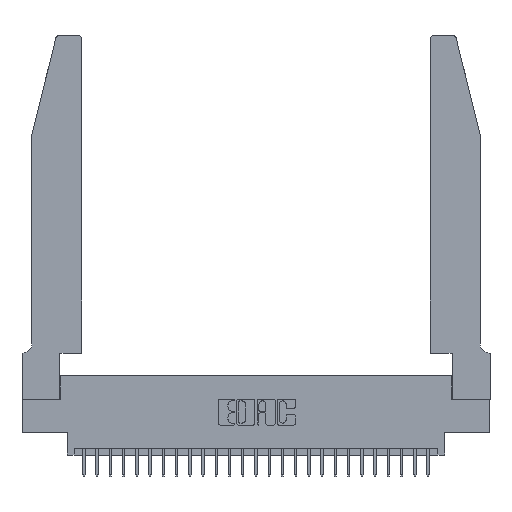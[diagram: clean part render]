
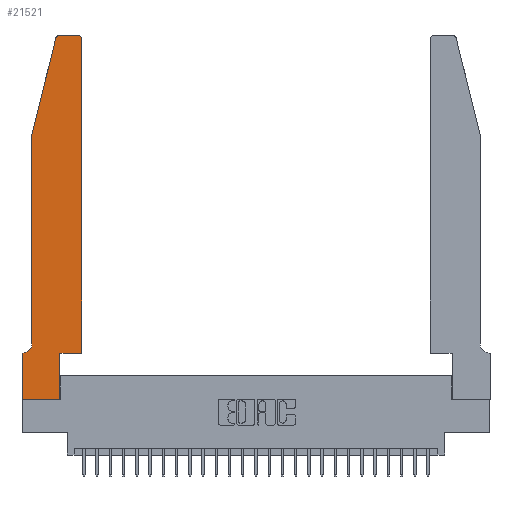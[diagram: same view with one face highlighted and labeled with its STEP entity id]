
A CAD part, top view. The second image highlights one B-rep face of the part: STEP entity #21521.
In plain terms, the highlighted planar face has unit normal (0, 0, 1).
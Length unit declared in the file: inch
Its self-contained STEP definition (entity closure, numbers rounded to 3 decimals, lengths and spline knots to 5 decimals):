
#35 = ORIENTED_EDGE ( 'NONE', *, *, #12355, .T. ) ;
#181 = CIRCLE ( 'NONE', #6082, 0.03 ) ;
#183 = CARTESIAN_POINT ( 'NONE',  ( 0.0755, 0.42, 0.37 ) ) ;
#223 = DIRECTION ( 'NONE',  ( 1., 0., 0. ) ) ;
#316 = CIRCLE ( 'NONE', #5066, 0.03 ) ;
#522 = VERTEX_POINT ( 'NONE', #19357 ) ;
#789 = ORIENTED_EDGE ( 'NONE', *, *, #21840, .T. ) ;
#815 = VECTOR ( 'NONE', #20764, 39.37008 ) ;
#1147 = CIRCLE ( 'NONE', #15072, 0.07 ) ;
#1433 = VECTOR ( 'NONE', #27402, 39.37008 ) ;
#1492 = LINE ( 'NONE', #7889, #815 ) ;
#1853 = CARTESIAN_POINT ( 'NONE',  ( 0.4505, 0.35, 0.37 ) ) ;
#1900 = VERTEX_POINT ( 'NONE', #2422 ) ;
#2214 = PLANE ( 'NONE',  #9395 ) ;
#2422 = CARTESIAN_POINT ( 'NONE',  ( 0.0755, 2., 0.37 ) ) ;
#2505 = DIRECTION ( 'NONE',  ( 0., 0., 1. ) ) ;
#2777 = VECTOR ( 'NONE', #16796, 39.37008 ) ;
#3103 = EDGE_CURVE ( 'NONE', #25998, #522, #1147, .T. ) ;
#3279 = DIRECTION ( 'NONE',  ( -1., 0., 0. ) ) ;
#3479 = DIRECTION ( 'NONE',  ( 1., 0., 0. ) ) ;
#3489 = LINE ( 'NONE', #9904, #1433 ) ;
#3537 = CARTESIAN_POINT ( 'NONE',  ( 0.25487, 2.72718, 0.37 ) ) ;
#3566 = DIRECTION ( 'NONE',  ( 0., 0., 1. ) ) ;
#3893 = LINE ( 'NONE', #26260, #12405 ) ;
#4237 = DIRECTION ( 'NONE',  ( -1., 0., 0. ) ) ;
#4612 = EDGE_CURVE ( 'NONE', #1900, #25998, #3489, .T. ) ;
#4697 = EDGE_CURVE ( 'NONE', #15780, #19619, #20827, .T. ) ;
#5066 = AXIS2_PLACEMENT_3D ( 'NONE', #10025, #3566, #27527 ) ;
#5402 = EDGE_LOOP ( 'NONE', ( #14896, #9479, #789, #10932, #7131, #21754, #7157, #11829, #24147, #20751, #17700, #35 ) ) ;
#5901 = VERTEX_POINT ( 'NONE', #23033 ) ;
#6082 = AXIS2_PLACEMENT_3D ( 'NONE', #6675, #19821, #223 ) ;
#6093 = CARTESIAN_POINT ( 'NONE',  ( 0.0755, 2., 0.37 ) ) ;
#6245 = CARTESIAN_POINT ( 'NONE',  ( 0.2865, 0.35, 0.37 ) ) ;
#6675 = CARTESIAN_POINT ( 'NONE',  ( 0.284, 2.72, 0.37 ) ) ;
#7131 = ORIENTED_EDGE ( 'NONE', *, *, #3103, .T. ) ;
#7157 = ORIENTED_EDGE ( 'NONE', *, *, #9062, .T. ) ;
#7889 = CARTESIAN_POINT ( 'NONE',  ( 0.0755, 0.35, 0.37 ) ) ;
#8300 = VERTEX_POINT ( 'NONE', #21572 ) ;
#8639 = VECTOR ( 'NONE', #14339, 39.37008 ) ;
#8862 = LINE ( 'NONE', #25642, #16047 ) ;
#9062 = EDGE_CURVE ( 'NONE', #14595, #8300, #3893, .T. ) ;
#9395 = AXIS2_PLACEMENT_3D ( 'NONE', #23641, #2505, #20128 ) ;
#9479 = ORIENTED_EDGE ( 'NONE', *, *, #21608, .T. ) ;
#9483 = EDGE_CURVE ( 'NONE', #19619, #17730, #19539, .T. ) ;
#9622 = VERTEX_POINT ( 'NONE', #22445 ) ;
#9625 = CARTESIAN_POINT ( 'NONE',  ( 0., 0.35, 0.37 ) ) ;
#9904 = CARTESIAN_POINT ( 'NONE',  ( 0.0755, 2., 0.37 ) ) ;
#10025 = CARTESIAN_POINT ( 'NONE',  ( 0.4205, 2.72, 0.37 ) ) ;
#10646 = CARTESIAN_POINT ( 'NONE',  ( 0.4505, 2.72, 0.37 ) ) ;
#10932 = ORIENTED_EDGE ( 'NONE', *, *, #4612, .T. ) ;
#11079 = LINE ( 'NONE', #6093, #16520 ) ;
#11829 = ORIENTED_EDGE ( 'NONE', *, *, #12826, .T. ) ;
#11856 = EDGE_CURVE ( 'NONE', #5901, #23019, #8862, .T. ) ;
#12043 = VECTOR ( 'NONE', #12820, 39.37008 ) ;
#12242 = CARTESIAN_POINT ( 'NONE',  ( 0.284, 2.75, 0.37 ) ) ;
#12355 = EDGE_CURVE ( 'NONE', #17730, #5901, #316, .T. ) ;
#12405 = VECTOR ( 'NONE', #14868, 39.37008 ) ;
#12820 = DIRECTION ( 'NONE',  ( 0., 1., 0. ) ) ;
#12826 = EDGE_CURVE ( 'NONE', #8300, #9622, #15642, .T. ) ;
#13456 = FACE_OUTER_BOUND ( 'NONE', #5402, .T. ) ;
#14339 = DIRECTION ( 'NONE',  ( 0., 1., 0. ) ) ;
#14595 = VERTEX_POINT ( 'NONE', #9625 ) ;
#14868 = DIRECTION ( 'NONE',  ( 0., -1., 0. ) ) ;
#14896 = ORIENTED_EDGE ( 'NONE', *, *, #11856, .T. ) ;
#15072 = AXIS2_PLACEMENT_3D ( 'NONE', #16237, #18396, #3279 ) ;
#15208 = CARTESIAN_POINT ( 'NONE',  ( 0.2865, 0.35, 0.37 ) ) ;
#15642 = LINE ( 'NONE', #25334, #24136 ) ;
#15780 = VERTEX_POINT ( 'NONE', #15208 ) ;
#16047 = VECTOR ( 'NONE', #4237, 39.37008 ) ;
#16237 = CARTESIAN_POINT ( 'NONE',  ( 0.0055, 0.42, 0.37 ) ) ;
#16419 = CARTESIAN_POINT ( 'NONE',  ( 0.4505, 0.35, 0.37 ) ) ;
#16520 = VECTOR ( 'NONE', #27245, 39.37008 ) ;
#16796 = DIRECTION ( 'NONE',  ( 1., 0., 0. ) ) ;
#17566 = VERTEX_POINT ( 'NONE', #3537 ) ;
#17700 = ORIENTED_EDGE ( 'NONE', *, *, #9483, .T. ) ;
#17730 = VERTEX_POINT ( 'NONE', #10646 ) ;
#18149 = LINE ( 'NONE', #6245, #12043 ) ;
#18396 = DIRECTION ( 'NONE',  ( 0., 0., -1. ) ) ;
#18860 = CARTESIAN_POINT ( 'NONE',  ( 0.4505, 0.35, 0.37 ) ) ;
#19357 = CARTESIAN_POINT ( 'NONE',  ( 0.0055, 0.35, 0.37 ) ) ;
#19539 = LINE ( 'NONE', #18860, #8639 ) ;
#19619 = VERTEX_POINT ( 'NONE', #16419 ) ;
#19821 = DIRECTION ( 'NONE',  ( 0., 0., 1. ) ) ;
#20128 = DIRECTION ( 'NONE',  ( 1., 0., 0. ) ) ;
#20751 = ORIENTED_EDGE ( 'NONE', *, *, #4697, .T. ) ;
#20764 = DIRECTION ( 'NONE',  ( -1., 0., 0. ) ) ;
#20827 = LINE ( 'NONE', #1853, #2777 ) ;
#21521 = ADVANCED_FACE ( 'NONE', ( #13456 ), #2214, .T. ) ;
#21572 = CARTESIAN_POINT ( 'NONE',  ( 0., 0., 0.37 ) ) ;
#21608 = EDGE_CURVE ( 'NONE', #23019, #17566, #181, .T. ) ;
#21754 = ORIENTED_EDGE ( 'NONE', *, *, #22236, .T. ) ;
#21840 = EDGE_CURVE ( 'NONE', #17566, #1900, #11079, .T. ) ;
#22236 = EDGE_CURVE ( 'NONE', #522, #14595, #1492, .T. ) ;
#22445 = CARTESIAN_POINT ( 'NONE',  ( 0.2865, 0., 0.37 ) ) ;
#22539 = EDGE_CURVE ( 'NONE', #9622, #15780, #18149, .T. ) ;
#23019 = VERTEX_POINT ( 'NONE', #12242 ) ;
#23033 = CARTESIAN_POINT ( 'NONE',  ( 0.4205, 2.75, 0.37 ) ) ;
#23641 = CARTESIAN_POINT ( 'NONE',  ( 0., 0.35, 0.37 ) ) ;
#24136 = VECTOR ( 'NONE', #3479, 39.37008 ) ;
#24147 = ORIENTED_EDGE ( 'NONE', *, *, #22539, .T. ) ;
#25334 = CARTESIAN_POINT ( 'NONE',  ( 0., 0., 0.37 ) ) ;
#25642 = CARTESIAN_POINT ( 'NONE',  ( 0.2605, 2.75, 0.37 ) ) ;
#25998 = VERTEX_POINT ( 'NONE', #183 ) ;
#26260 = CARTESIAN_POINT ( 'NONE',  ( 0., 0., 0.37 ) ) ;
#27245 = DIRECTION ( 'NONE',  ( -0.239, -0.971, 0. ) ) ;
#27402 = DIRECTION ( 'NONE',  ( 0., -1., 0. ) ) ;
#27527 = DIRECTION ( 'NONE',  ( 1., 0., 0. ) ) ;
